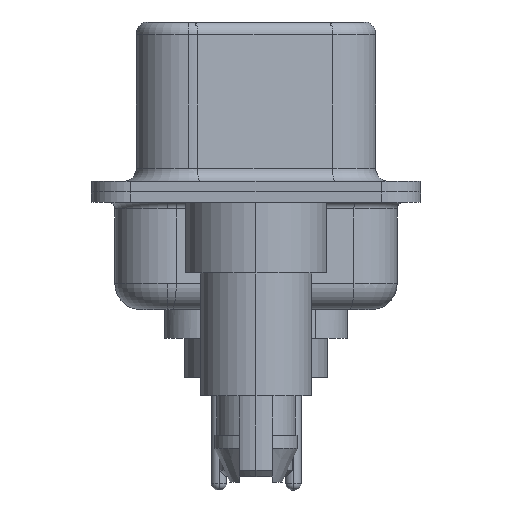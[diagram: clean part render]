
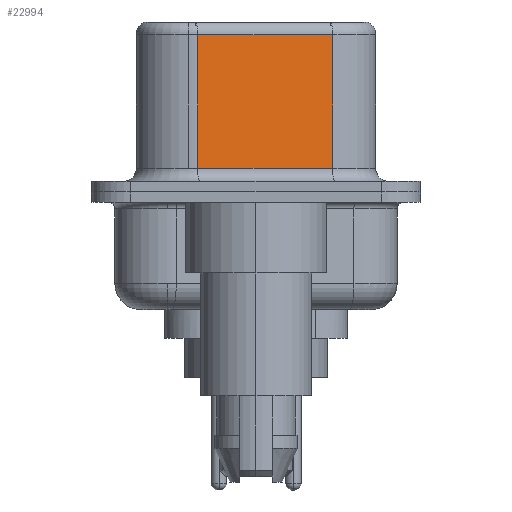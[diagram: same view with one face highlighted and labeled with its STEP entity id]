
A CAD part, left-side view. The second image highlights one B-rep face of the part: STEP entity #22994.
In plain terms, the highlighted planar face has unit normal (-0.985, -0.174, 0).
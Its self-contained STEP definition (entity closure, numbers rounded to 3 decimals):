
#641 = LINE ( 'NONE', #17077, #16386 ) ;
#937 = LINE ( 'NONE', #22669, #5718 ) ;
#1044 = ORIENTED_EDGE ( 'NONE', *, *, #8972, .T. ) ;
#1735 = CARTESIAN_POINT ( 'NONE',  ( 4.58, -2.927, 6.52 ) ) ;
#1742 = FACE_OUTER_BOUND ( 'NONE', #8536, .T. ) ;
#1849 = VERTEX_POINT ( 'NONE', #14718 ) ;
#2720 = VECTOR ( 'NONE', #14080, 1000. ) ;
#2842 = DIRECTION ( 'NONE',  ( 0.174, -0.985, 0. ) ) ;
#3510 = ORIENTED_EDGE ( 'NONE', *, *, #11135, .F. ) ;
#5718 = VECTOR ( 'NONE', #20740, 1000. ) ;
#8098 = ORIENTED_EDGE ( 'NONE', *, *, #18562, .T. ) ;
#8177 = LINE ( 'NONE', #1735, #2720 ) ;
#8536 = EDGE_LOOP ( 'NONE', ( #3510, #22223, #1044, #8098 ) ) ;
#8750 = VECTOR ( 'NONE', #12660, 1000. ) ;
#8972 = EDGE_CURVE ( 'NONE', #17314, #22302, #937, .T. ) ;
#10326 = CARTESIAN_POINT ( 'NONE',  ( 4.58, -2.927, 6.02 ) ) ;
#10506 = CARTESIAN_POINT ( 'NONE',  ( 4.58, -2.927, 6.52 ) ) ;
#10563 = CARTESIAN_POINT ( 'NONE',  ( 4.58, -2.927, 6.02 ) ) ;
#10619 = CARTESIAN_POINT ( 'NONE',  ( 3.67, 2.233, 0.9 ) ) ;
#10683 = DIRECTION ( 'NONE',  ( 0.985, 0.174, 0. ) ) ;
#11135 = EDGE_CURVE ( 'NONE', #14076, #1849, #8177, .T. ) ;
#12660 = DIRECTION ( 'NONE',  ( -0.174, 0.985, 0. ) ) ;
#14076 = VERTEX_POINT ( 'NONE', #10326 ) ;
#14080 = DIRECTION ( 'NONE',  ( 0., 0., -1. ) ) ;
#14718 = CARTESIAN_POINT ( 'NONE',  ( 4.58, -2.927, 0.9 ) ) ;
#16386 = VECTOR ( 'NONE', #2842, 1000. ) ;
#17077 = CARTESIAN_POINT ( 'NONE',  ( 4.58, -2.927, 0.9 ) ) ;
#17314 = VERTEX_POINT ( 'NONE', #23651 ) ;
#18562 = EDGE_CURVE ( 'NONE', #22302, #1849, #641, .T. ) ;
#18801 = AXIS2_PLACEMENT_3D ( 'NONE', #10506, #10683, #24955 ) ;
#20740 = DIRECTION ( 'NONE',  ( 0., 0., -1. ) ) ;
#20881 = PLANE ( 'NONE',  #18801 ) ;
#22223 = ORIENTED_EDGE ( 'NONE', *, *, #23623, .T. ) ;
#22302 = VERTEX_POINT ( 'NONE', #10619 ) ;
#22669 = CARTESIAN_POINT ( 'NONE',  ( 3.67, 2.233, 6.52 ) ) ;
#22994 = ADVANCED_FACE ( 'NONE', ( #1742 ), #20881, .F. ) ;
#23623 = EDGE_CURVE ( 'NONE', #14076, #17314, #24432, .T. ) ;
#23651 = CARTESIAN_POINT ( 'NONE',  ( 3.67, 2.233, 6.02 ) ) ;
#24432 = LINE ( 'NONE', #10563, #8750 ) ;
#24955 = DIRECTION ( 'NONE',  ( -0.174, 0.985, 0. ) ) ;
